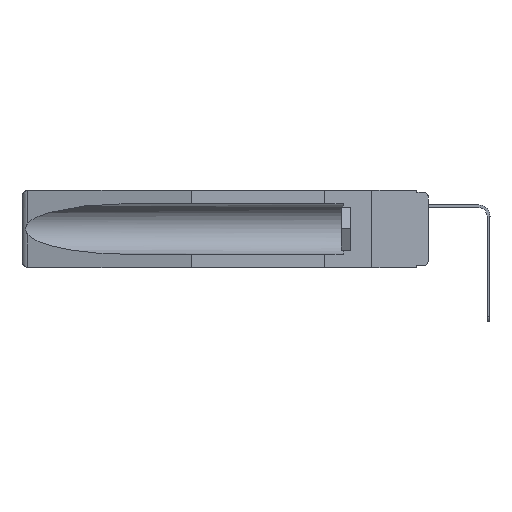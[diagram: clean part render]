
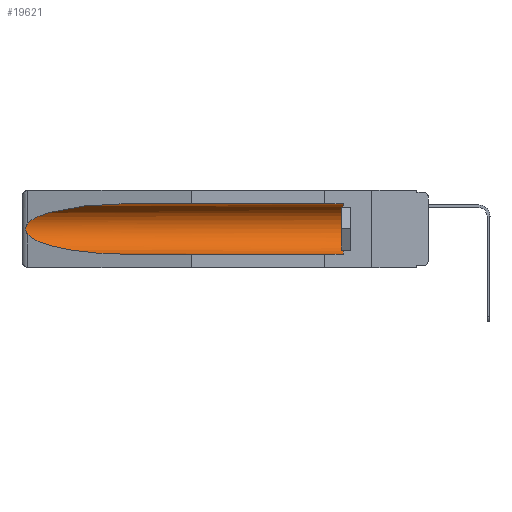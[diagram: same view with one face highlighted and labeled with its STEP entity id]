
A CAD part, left-side view. The second image highlights one B-rep face of the part: STEP entity #19621.
In plain terms, the highlighted cylindrical face has radius 2.857 mm (diameter 5.715 mm), a partial arc.
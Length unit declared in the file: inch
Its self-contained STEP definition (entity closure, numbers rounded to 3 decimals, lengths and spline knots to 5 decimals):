
#1260 = VERTEX_POINT ( 'NONE', #17816 ) ;
#2299 = CARTESIAN_POINT ( 'NONE',  ( 0.26537, 1.52718, -0.14972 ) ) ;
#2670 = CARTESIAN_POINT ( 'NONE',  ( 0.155, -0.30754, -0.284 ) ) ;
#3117 = CARTESIAN_POINT ( 'NONE',  ( 0.26537, 1.52718, -0.19328 ) ) ;
#3209 = CARTESIAN_POINT ( 'NONE',  ( 0.2675, 1.53308, -0.16763 ) ) ;
#3685 = B_SPLINE_CURVE_WITH_KNOTS ( 'NONE', 3,
 ( #7259, #6990, #23075, #9294, #3209, #5059, #11127, #21052, #15173, #3117 ),
 .UNSPECIFIED., .F., .F.,
 ( 4, 2, 2, 2, 4 ),
 ( 0., 0.00029, 0.00058, 0.00087, 0.00117 ),
 .UNSPECIFIED. ) ;
#4373 = CARTESIAN_POINT ( 'NONE',  ( 0.155, 0.126, -0.284 ) ) ;
#4604 = ORIENTED_EDGE ( 'NONE', *, *, #18034, .F. ) ;
#5059 = CARTESIAN_POINT ( 'NONE',  ( 0.2675, 1.53308, -0.17534 ) ) ;
#5775 = EDGE_CURVE ( 'NONE', #6900, #24817, #3685, .T. ) ;
#5900 = ORIENTED_EDGE ( 'NONE', *, *, #12144, .T. ) ;
#6462 = DIRECTION ( 'NONE',  ( 0., -1., 0. ) ) ;
#6542 = CARTESIAN_POINT ( 'NONE',  ( 0.155, 0.126, -0.1715 ) ) ;
#6900 = VERTEX_POINT ( 'NONE', #20405 ) ;
#6990 = CARTESIAN_POINT ( 'NONE',  ( 0.26597, 1.52961, -0.15275 ) ) ;
#7014 = CARTESIAN_POINT ( 'NONE',  ( 0.155, 1.07973, -0.284 ) ) ;
#7259 = CARTESIAN_POINT ( 'NONE',  ( 0.26537, 1.52718, -0.14972 ) ) ;
#7465 = LINE ( 'NONE', #2670, #13719 ) ;
#7505 = CIRCLE ( 'NONE', #16190, 0.1125 ) ;
#8223 = CARTESIAN_POINT ( 'NONE',  ( 0.21114, 1.30732, -0.059 ) ) ;
#8487 = CARTESIAN_POINT ( 'NONE',  ( 0.155, 1.07973, -0.059 ) ) ;
#9294 = CARTESIAN_POINT ( 'NONE',  ( 0.2673, 1.5327, -0.16383 ) ) ;
#9428 = CARTESIAN_POINT ( 'NONE',  ( 0.155, -0.30754, -0.059 ) ) ;
#9718 = VERTEX_POINT ( 'NONE', #16464 ) ;
#10089 = ORIENTED_EDGE ( 'NONE', *, *, #10430, .T. ) ;
#10430 = EDGE_CURVE ( 'NONE', #24817, #9718, #20472, .T. ) ;
#11059 = CARTESIAN_POINT ( 'NONE',  ( 0.26537, 1.52718, -0.19328 ) ) ;
#11127 = CARTESIAN_POINT ( 'NONE',  ( 0.2673, 1.53269, -0.17917 ) ) ;
#11536 = CARTESIAN_POINT ( 'NONE',  ( 0.26537, 1.52718, -0.19328 ) ) ;
#12104 = ORIENTED_EDGE ( 'NONE', *, *, #17125, .T. ) ;
#12144 = EDGE_CURVE ( 'NONE', #1260, #6900, #15788, .T. ) ;
#12283 = VECTOR ( 'NONE', #17588, 39.37008 ) ;
#12591 = ORIENTED_EDGE ( 'NONE', *, *, #5775, .T. ) ;
#12696 = DIRECTION ( 'NONE',  ( 0., 1., 0. ) ) ;
#13707 = EDGE_LOOP ( 'NONE', ( #5900, #12591, #10089, #4604, #12104, #16262 ) ) ;
#13719 = VECTOR ( 'NONE', #12696, 39.37008 ) ;
#13932 = CARTESIAN_POINT ( 'NONE',  ( 0.155, 0.126, -0.059 ) ) ;
#14296 = CARTESIAN_POINT ( 'NONE',  ( 0.155, -0.30754, -0.1715 ) ) ;
#14591 = AXIS2_PLACEMENT_3D ( 'NONE', #14296, #20449, #20357 ) ;
#14937 = CARTESIAN_POINT ( 'NONE',  ( 0.25451, 1.48313, -0.24835 ) ) ;
#15173 = CARTESIAN_POINT ( 'NONE',  ( 0.26597, 1.5296, -0.19026 ) ) ;
#15644 = EDGE_CURVE ( 'NONE', #26086, #1260, #17630, .T. ) ;
#15788 =( BOUNDED_CURVE ( )  B_SPLINE_CURVE ( 3, ( #8487, #8223, #24366, #2299 ),
 .UNSPECIFIED., .F., .T. ) 
 B_SPLINE_CURVE_WITH_KNOTS ( ( 4, 4 ),
 ( 4.71239, 6.08839 ),
 .UNSPECIFIED. ) 
 CURVE ( )  GEOMETRIC_REPRESENTATION_ITEM ( )  RATIONAL_B_SPLINE_CURVE ( ( 1., 0.848, 0.848, 1. ) ) 
 REPRESENTATION_ITEM ( '' )  );
#16190 = AXIS2_PLACEMENT_3D ( 'NONE', #6542, #6462, #22539 ) ;
#16262 = ORIENTED_EDGE ( 'NONE', *, *, #15644, .T. ) ;
#16464 = CARTESIAN_POINT ( 'NONE',  ( 0.155, 1.07973, -0.284 ) ) ;
#17125 = EDGE_CURVE ( 'NONE', #23828, #26086, #7505, .T. ) ;
#17588 = DIRECTION ( 'NONE',  ( 0., 1., 0. ) ) ;
#17630 = LINE ( 'NONE', #9428, #12283 ) ;
#17816 = CARTESIAN_POINT ( 'NONE',  ( 0.155, 1.07973, -0.059 ) ) ;
#18034 = EDGE_CURVE ( 'NONE', #23828, #9718, #7465, .T. ) ;
#18884 = CARTESIAN_POINT ( 'NONE',  ( 0.21114, 1.30732, -0.284 ) ) ;
#19621 = ADVANCED_FACE ( 'NONE', ( #20666 ), #20032, .F. ) ;
#20032 = CYLINDRICAL_SURFACE ( 'NONE', #14591, 0.1125 ) ;
#20357 = DIRECTION ( 'NONE',  ( 0., 0., 1. ) ) ;
#20405 = CARTESIAN_POINT ( 'NONE',  ( 0.26537, 1.52718, -0.14972 ) ) ;
#20449 = DIRECTION ( 'NONE',  ( 0., 1., 0. ) ) ;
#20472 =( BOUNDED_CURVE ( )  B_SPLINE_CURVE ( 3, ( #11059, #14937, #18884, #7014 ),
 .UNSPECIFIED., .F., .F. ) 
 B_SPLINE_CURVE_WITH_KNOTS ( ( 4, 4 ),
 ( 0.1948, 1.5708 ),
 .UNSPECIFIED. ) 
 CURVE ( )  GEOMETRIC_REPRESENTATION_ITEM ( )  RATIONAL_B_SPLINE_CURVE ( ( 1., 0.848, 0.848, 1. ) ) 
 REPRESENTATION_ITEM ( '' )  );
#20666 = FACE_OUTER_BOUND ( 'NONE', #13707, .T. ) ;
#21052 = CARTESIAN_POINT ( 'NONE',  ( 0.26655, 1.53094, -0.18657 ) ) ;
#22539 = DIRECTION ( 'NONE',  ( 0., 0., 1. ) ) ;
#23075 = CARTESIAN_POINT ( 'NONE',  ( 0.26654, 1.53092, -0.15636 ) ) ;
#23828 = VERTEX_POINT ( 'NONE', #4373 ) ;
#24366 = CARTESIAN_POINT ( 'NONE',  ( 0.25451, 1.48313, -0.09465 ) ) ;
#24817 = VERTEX_POINT ( 'NONE', #11536 ) ;
#26086 = VERTEX_POINT ( 'NONE', #13932 ) ;
